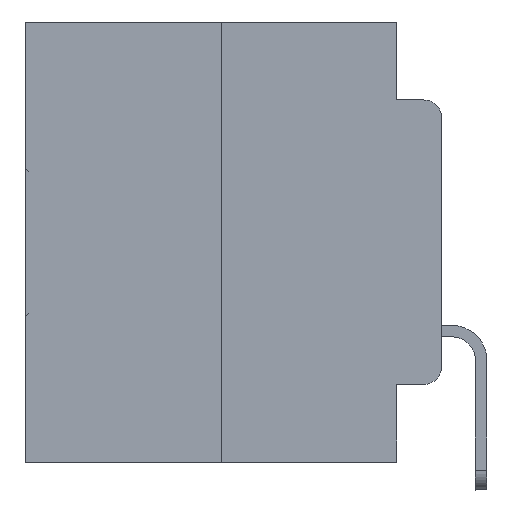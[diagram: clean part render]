
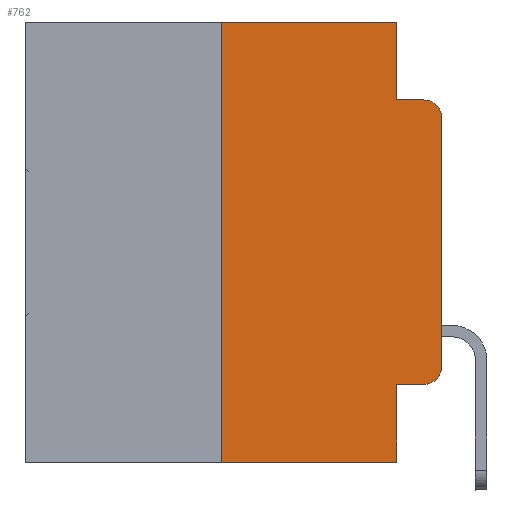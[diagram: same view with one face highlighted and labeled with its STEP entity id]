
A CAD part, left-side view. The second image highlights one B-rep face of the part: STEP entity #762.
In plain terms, the highlighted planar face has unit normal (-1, 0, 0).
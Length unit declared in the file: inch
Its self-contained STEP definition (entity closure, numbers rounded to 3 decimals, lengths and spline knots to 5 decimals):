
#451 = ORIENTED_EDGE ( 'NONE', *, *, #18337, .T. ) ;
#762 = ADVANCED_FACE ( 'NONE', ( #7214 ), #7499, .F. ) ;
#1098 = EDGE_CURVE ( 'NONE', #3776, #18156, #4362, .T. ) ;
#1884 = ORIENTED_EDGE ( 'NONE', *, *, #21427, .T. ) ;
#2476 = LINE ( 'NONE', #14377, #25149 ) ;
#2596 = EDGE_LOOP ( 'NONE', ( #2666, #451, #19358, #14339, #28169, #22506, #25222, #8576, #20801, #1884 ) ) ;
#2666 = ORIENTED_EDGE ( 'NONE', *, *, #17131, .T. ) ;
#2691 = EDGE_CURVE ( 'NONE', #3776, #12850, #11884, .T. ) ;
#3422 = VECTOR ( 'NONE', #13814, 39.37008 ) ;
#3487 = CIRCLE ( 'NONE', #6803, 0.02 ) ;
#3776 = VERTEX_POINT ( 'NONE', #23633 ) ;
#4073 = CARTESIAN_POINT ( 'NONE',  ( 0., 0.051, -0.4115 ) ) ;
#4121 = CARTESIAN_POINT ( 'NONE',  ( 0., 0.02, -0.0885 ) ) ;
#4362 = LINE ( 'NONE', #17645, #28372 ) ;
#4769 = VECTOR ( 'NONE', #5029, 39.37008 ) ;
#5029 = DIRECTION ( 'NONE',  ( 0., 0., 1. ) ) ;
#5393 = CARTESIAN_POINT ( 'NONE',  ( 0., 0.473, 0. ) ) ;
#5625 = CARTESIAN_POINT ( 'NONE',  ( 0., 0.25, 0. ) ) ;
#6707 = DIRECTION ( 'NONE',  ( -1., 0., 0. ) ) ;
#6803 = AXIS2_PLACEMENT_3D ( 'NONE', #15623, #13834, #20412 ) ;
#6816 = LINE ( 'NONE', #13954, #3422 ) ;
#6952 = EDGE_CURVE ( 'NONE', #27542, #18156, #2476, .T. ) ;
#7214 = FACE_OUTER_BOUND ( 'NONE', #2596, .T. ) ;
#7499 = PLANE ( 'NONE',  #11153 ) ;
#7775 = DIRECTION ( 'NONE',  ( 0., -1., 0. ) ) ;
#7791 = CARTESIAN_POINT ( 'NONE',  ( 0., 0.473, 0. ) ) ;
#8464 = VERTEX_POINT ( 'NONE', #14420 ) ;
#8576 = ORIENTED_EDGE ( 'NONE', *, *, #6952, .F. ) ;
#8668 = DIRECTION ( 'NONE',  ( 0., -1., 0. ) ) ;
#8760 = CARTESIAN_POINT ( 'NONE',  ( 0., 0.051, -0.0885 ) ) ;
#8910 = CARTESIAN_POINT ( 'NONE',  ( 0., 0.02, -0.1085 ) ) ;
#9008 = VECTOR ( 'NONE', #24632, 39.37008 ) ;
#9240 = VERTEX_POINT ( 'NONE', #23745 ) ;
#9343 = CARTESIAN_POINT ( 'NONE',  ( 0., 0., 0. ) ) ;
#9443 = VERTEX_POINT ( 'NONE', #8760 ) ;
#9544 = VERTEX_POINT ( 'NONE', #11734 ) ;
#9704 = DIRECTION ( 'NONE',  ( 1., 0., 0. ) ) ;
#10118 = CARTESIAN_POINT ( 'NONE',  ( 0., 0.051, -0.4115 ) ) ;
#11153 = AXIS2_PLACEMENT_3D ( 'NONE', #7791, #9704, #25437 ) ;
#11544 = DIRECTION ( 'NONE',  ( 0., 0., -1. ) ) ;
#11734 = CARTESIAN_POINT ( 'NONE',  ( 0., 0.02, -0.4115 ) ) ;
#11884 = LINE ( 'NONE', #25796, #16432 ) ;
#12464 = VECTOR ( 'NONE', #8668, 39.37008 ) ;
#12660 = CARTESIAN_POINT ( 'NONE',  ( 0., 0.051, -0.5 ) ) ;
#12850 = VERTEX_POINT ( 'NONE', #5625 ) ;
#13452 = DIRECTION ( 'NONE',  ( 0., -1., 0. ) ) ;
#13814 = DIRECTION ( 'NONE',  ( 0., 0., -1. ) ) ;
#13834 = DIRECTION ( 'NONE',  ( -1., 0., 0. ) ) ;
#13954 = CARTESIAN_POINT ( 'NONE',  ( 0., 0.051, 0. ) ) ;
#14339 = ORIENTED_EDGE ( 'NONE', *, *, #18733, .F. ) ;
#14377 = CARTESIAN_POINT ( 'NONE',  ( 0., 0.051, 0. ) ) ;
#14420 = CARTESIAN_POINT ( 'NONE',  ( 0., 0.051, 0. ) ) ;
#15395 = LINE ( 'NONE', #4073, #12464 ) ;
#15623 = CARTESIAN_POINT ( 'NONE',  ( 0., 0.02, -0.3915 ) ) ;
#16432 = VECTOR ( 'NONE', #19063, 39.37008 ) ;
#16604 = EDGE_CURVE ( 'NONE', #12850, #8464, #26319, .T. ) ;
#17131 = EDGE_CURVE ( 'NONE', #25695, #9240, #18173, .T. ) ;
#17430 = VERTEX_POINT ( 'NONE', #4121 ) ;
#17645 = CARTESIAN_POINT ( 'NONE',  ( 0., 0.473, -0.5 ) ) ;
#18148 = AXIS2_PLACEMENT_3D ( 'NONE', #8910, #6707, #28953 ) ;
#18156 = VERTEX_POINT ( 'NONE', #12660 ) ;
#18173 = LINE ( 'NONE', #9343, #4769 ) ;
#18337 = EDGE_CURVE ( 'NONE', #9240, #17430, #21506, .T. ) ;
#18617 = CARTESIAN_POINT ( 'NONE',  ( 0., 0., -0.3915 ) ) ;
#18733 = EDGE_CURVE ( 'NONE', #8464, #9443, #6816, .T. ) ;
#19063 = DIRECTION ( 'NONE',  ( 0., 0., 1. ) ) ;
#19135 = EDGE_CURVE ( 'NONE', #27542, #9544, #15395, .T. ) ;
#19358 = ORIENTED_EDGE ( 'NONE', *, *, #29021, .F. ) ;
#20412 = DIRECTION ( 'NONE',  ( 0., 0., -1. ) ) ;
#20801 = ORIENTED_EDGE ( 'NONE', *, *, #19135, .T. ) ;
#21417 = VECTOR ( 'NONE', #7775, 39.37008 ) ;
#21427 = EDGE_CURVE ( 'NONE', #9544, #25695, #3487, .T. ) ;
#21506 = CIRCLE ( 'NONE', #18148, 0.02 ) ;
#22506 = ORIENTED_EDGE ( 'NONE', *, *, #2691, .F. ) ;
#22994 = LINE ( 'NONE', #29116, #9008 ) ;
#23633 = CARTESIAN_POINT ( 'NONE',  ( 0., 0.25, -0.5 ) ) ;
#23745 = CARTESIAN_POINT ( 'NONE',  ( 0., 0., -0.1085 ) ) ;
#24632 = DIRECTION ( 'NONE',  ( 0., -1., 0. ) ) ;
#25149 = VECTOR ( 'NONE', #11544, 39.37008 ) ;
#25222 = ORIENTED_EDGE ( 'NONE', *, *, #1098, .T. ) ;
#25437 = DIRECTION ( 'NONE',  ( 0., 0., -1. ) ) ;
#25695 = VERTEX_POINT ( 'NONE', #18617 ) ;
#25796 = CARTESIAN_POINT ( 'NONE',  ( 0., 0.25, 0. ) ) ;
#26319 = LINE ( 'NONE', #5393, #21417 ) ;
#27542 = VERTEX_POINT ( 'NONE', #10118 ) ;
#28169 = ORIENTED_EDGE ( 'NONE', *, *, #16604, .F. ) ;
#28372 = VECTOR ( 'NONE', #13452, 39.37008 ) ;
#28953 = DIRECTION ( 'NONE',  ( 0., 0., -1. ) ) ;
#29021 = EDGE_CURVE ( 'NONE', #9443, #17430, #22994, .T. ) ;
#29116 = CARTESIAN_POINT ( 'NONE',  ( 0., 0.051, -0.0885 ) ) ;
